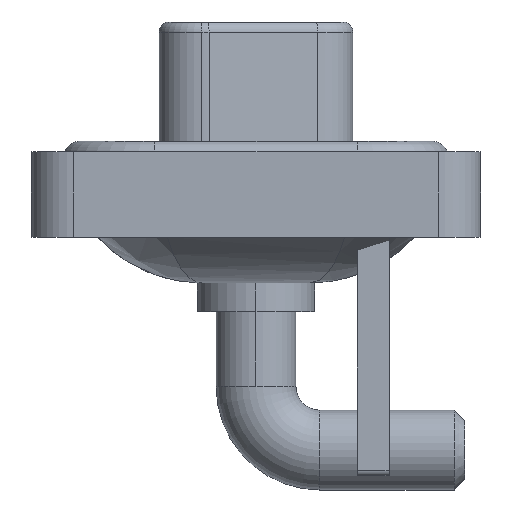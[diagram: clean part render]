
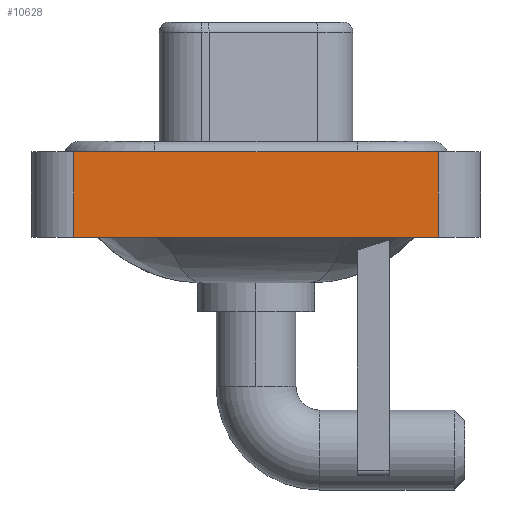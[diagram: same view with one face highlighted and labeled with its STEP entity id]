
A CAD part, left-side view. The second image highlights one B-rep face of the part: STEP entity #10628.
In plain terms, the highlighted planar face has unit normal (-1, 0, 0).
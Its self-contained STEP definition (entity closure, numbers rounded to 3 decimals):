
#152 = DIRECTION ( 'NONE',  ( 0., -1., 0. ) ) ;
#359 = DIRECTION ( 'NONE',  ( 0., -1., 0. ) ) ;
#1615 = AXIS2_PLACEMENT_3D ( 'NONE', #9150, #12822, #12084 ) ;
#2614 = LINE ( 'NONE', #2693, #9593 ) ;
#2678 = LINE ( 'NONE', #9987, #9817 ) ;
#2693 = CARTESIAN_POINT ( 'NONE',  ( -7.25, -8.55, -3.6 ) ) ;
#2703 = VERTEX_POINT ( 'NONE', #7148 ) ;
#3497 = EDGE_CURVE ( 'NONE', #10494, #15011, #11207, .T. ) ;
#4080 = CARTESIAN_POINT ( 'NONE',  ( -7.25, 8.55, -3.6 ) ) ;
#5025 = CARTESIAN_POINT ( 'NONE',  ( -7.25, 8.55, 0.4 ) ) ;
#5890 = CARTESIAN_POINT ( 'NONE',  ( -7.25, -8.55, -3.6 ) ) ;
#5982 = FACE_OUTER_BOUND ( 'NONE', #13599, .T. ) ;
#7148 = CARTESIAN_POINT ( 'NONE',  ( -7.25, -8.55, 0.4 ) ) ;
#7155 = VECTOR ( 'NONE', #152, 1000. ) ;
#7161 = EDGE_CURVE ( 'NONE', #15011, #2703, #14979, .T. ) ;
#7541 = CARTESIAN_POINT ( 'NONE',  ( -7.25, 8.55, -3.6 ) ) ;
#8374 = VECTOR ( 'NONE', #14461, 1000. ) ;
#9122 = VERTEX_POINT ( 'NONE', #5890 ) ;
#9150 = CARTESIAN_POINT ( 'NONE',  ( -7.25, -8.55, -3.6 ) ) ;
#9593 = VECTOR ( 'NONE', #359, 1000. ) ;
#9817 = VECTOR ( 'NONE', #14870, 1000. ) ;
#9987 = CARTESIAN_POINT ( 'NONE',  ( -7.25, -8.55, -3.6 ) ) ;
#10494 = VERTEX_POINT ( 'NONE', #4080 ) ;
#10628 = ADVANCED_FACE ( 'NONE', ( #5982 ), #11624, .T. ) ;
#11167 = ORIENTED_EDGE ( 'NONE', *, *, #13683, .T. ) ;
#11207 = LINE ( 'NONE', #7541, #8374 ) ;
#11214 = CARTESIAN_POINT ( 'NONE',  ( -7.25, -8.55, 0.4 ) ) ;
#11624 = PLANE ( 'NONE',  #1615 ) ;
#12084 = DIRECTION ( 'NONE',  ( 0., 0., 1. ) ) ;
#12822 = DIRECTION ( 'NONE',  ( -1., 0., 0. ) ) ;
#13599 = EDGE_LOOP ( 'NONE', ( #11167, #15351, #14736, #14560 ) ) ;
#13683 = EDGE_CURVE ( 'NONE', #9122, #2703, #2678, .T. ) ;
#14461 = DIRECTION ( 'NONE',  ( 0., 0., 1. ) ) ;
#14560 = ORIENTED_EDGE ( 'NONE', *, *, #15085, .T. ) ;
#14736 = ORIENTED_EDGE ( 'NONE', *, *, #3497, .F. ) ;
#14870 = DIRECTION ( 'NONE',  ( 0., 0., 1. ) ) ;
#14979 = LINE ( 'NONE', #11214, #7155 ) ;
#15011 = VERTEX_POINT ( 'NONE', #5025 ) ;
#15085 = EDGE_CURVE ( 'NONE', #10494, #9122, #2614, .T. ) ;
#15351 = ORIENTED_EDGE ( 'NONE', *, *, #7161, .F. ) ;
